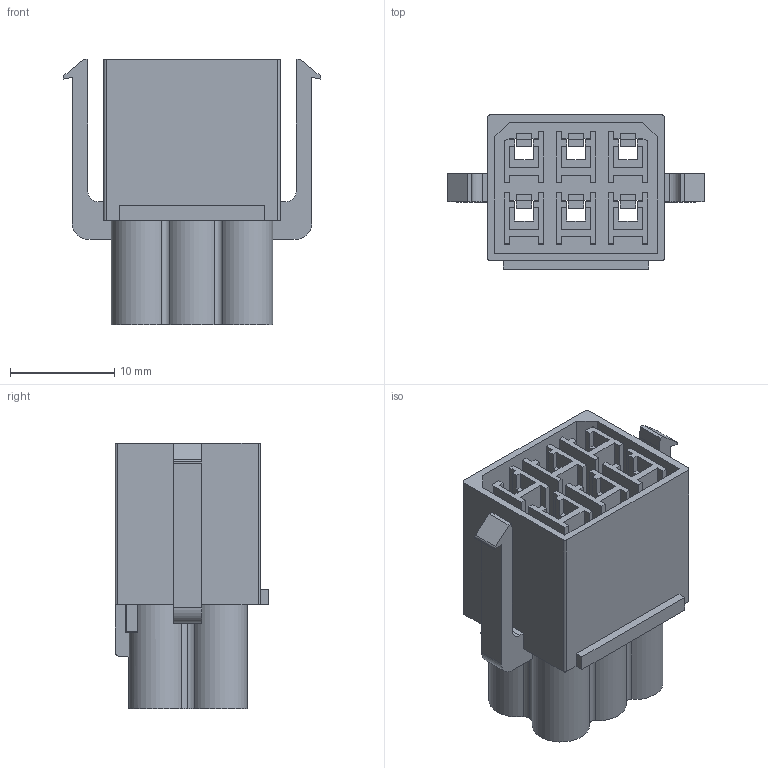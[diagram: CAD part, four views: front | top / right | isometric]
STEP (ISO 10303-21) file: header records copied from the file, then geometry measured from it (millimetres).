
FILE_DESCRIPTION (( 'STEP AP214' ), '1' );
FILE_NAME ('567-006-000-410.STEP', '2020-07-27T20:17:26', ( '' ), ( '' ), 'SwSTEP 2.0', 'SolidWorks 2020', '' );
FILE_SCHEMA (( 'AUTOMOTIVE_DESIGN' ));
Length unit declared in the file: millimetre
Products named in the file (1): 567-006-000-410
Bounding box: 24.8 x 14.8 x 25.5 mm (x, y, z)
Volume: 2223.2 mm3; surface area: 6610.1 mm2
Topology: 1 solids, 1 shells, 489 faces, 1391 edges, 920 vertices
Faces by surface type: plane 394, cylinder 72, bspline 21, sphere 2
Entity records: 16801 total; most frequent: CARTESIAN_POINT 4124, ORIENTED_EDGE 2778, DIRECTION 2405, EDGE_CURVE 1389, LINE 1151, VECTOR 1151, VERTEX_POINT 920, AXIS2_PLACEMENT_3D 627
